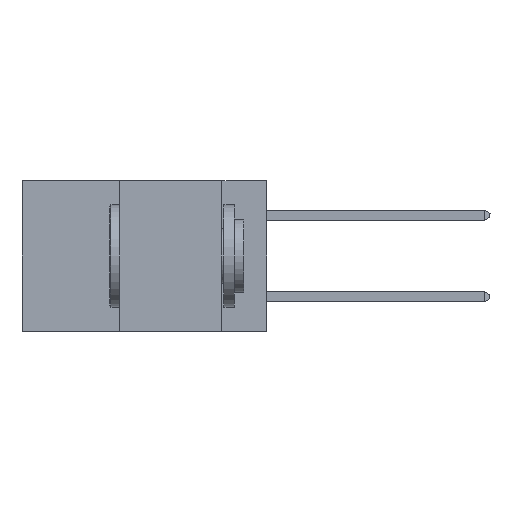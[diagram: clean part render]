
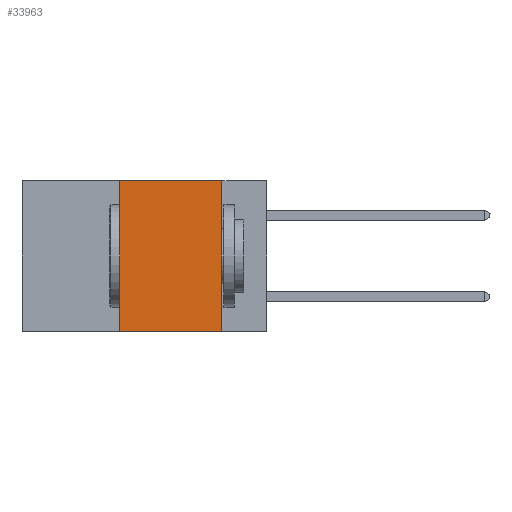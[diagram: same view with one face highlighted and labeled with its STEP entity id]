
A CAD part, left-side view. The second image highlights one B-rep face of the part: STEP entity #33963.
In plain terms, the highlighted planar face has unit normal (-1, 0, 0).
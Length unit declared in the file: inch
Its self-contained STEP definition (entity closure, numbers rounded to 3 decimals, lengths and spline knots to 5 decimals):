
#329 = CARTESIAN_POINT ( 'NONE',  ( 0., 0.6, 0. ) ) ;
#788 = DIRECTION ( 'NONE',  ( 0., 0., 1. ) ) ;
#1015 = CARTESIAN_POINT ( 'NONE',  ( 0., 0.6, 0. ) ) ;
#2139 = CARTESIAN_POINT ( 'NONE',  ( 0., 0.11, -0.37 ) ) ;
#2255 = LINE ( 'NONE', #22179, #9392 ) ;
#3191 = DIRECTION ( 'NONE',  ( 0., -1., 0. ) ) ;
#6124 = DIRECTION ( 'NONE',  ( 0., -1., 0. ) ) ;
#6449 = PLANE ( 'NONE',  #34314 ) ;
#6854 = ORIENTED_EDGE ( 'NONE', *, *, #11763, .F. ) ;
#8208 = EDGE_LOOP ( 'NONE', ( #16887, #12292, #6854, #29658 ) ) ;
#8418 = FACE_OUTER_BOUND ( 'NONE', #8208, .T. ) ;
#8874 = CARTESIAN_POINT ( 'NONE',  ( 0., 0.36, -0.37 ) ) ;
#9163 = DIRECTION ( 'NONE',  ( 1., 0., 0. ) ) ;
#9392 = VECTOR ( 'NONE', #788, 39.37008 ) ;
#10260 = LINE ( 'NONE', #329, #15704 ) ;
#11763 = EDGE_CURVE ( 'NONE', #21095, #29034, #2255, .T. ) ;
#11818 = LINE ( 'NONE', #25637, #25072 ) ;
#12292 = ORIENTED_EDGE ( 'NONE', *, *, #27931, .F. ) ;
#14019 = VECTOR ( 'NONE', #6124, 39.37008 ) ;
#14948 = VERTEX_POINT ( 'NONE', #26959 ) ;
#15704 = VECTOR ( 'NONE', #3191, 39.37008 ) ;
#15871 = VERTEX_POINT ( 'NONE', #2139 ) ;
#16887 = ORIENTED_EDGE ( 'NONE', *, *, #19575, .F. ) ;
#19575 = EDGE_CURVE ( 'NONE', #14948, #15871, #11818, .T. ) ;
#21095 = VERTEX_POINT ( 'NONE', #8874 ) ;
#22083 = CARTESIAN_POINT ( 'NONE',  ( 0., 0.6, -0.37 ) ) ;
#22179 = CARTESIAN_POINT ( 'NONE',  ( 0., 0.36, 0. ) ) ;
#25072 = VECTOR ( 'NONE', #30793, 39.37008 ) ;
#25637 = CARTESIAN_POINT ( 'NONE',  ( 0., 0.11, 0. ) ) ;
#26959 = CARTESIAN_POINT ( 'NONE',  ( 0., 0.11, 0. ) ) ;
#27678 = DIRECTION ( 'NONE',  ( 0., 0., -1. ) ) ;
#27931 = EDGE_CURVE ( 'NONE', #29034, #14948, #10260, .T. ) ;
#27991 = EDGE_CURVE ( 'NONE', #21095, #15871, #34240, .T. ) ;
#29034 = VERTEX_POINT ( 'NONE', #31981 ) ;
#29658 = ORIENTED_EDGE ( 'NONE', *, *, #27991, .T. ) ;
#30793 = DIRECTION ( 'NONE',  ( 0., 0., -1. ) ) ;
#31981 = CARTESIAN_POINT ( 'NONE',  ( 0., 0.36, 0. ) ) ;
#33963 = ADVANCED_FACE ( 'NONE', ( #8418 ), #6449, .F. ) ;
#34240 = LINE ( 'NONE', #22083, #14019 ) ;
#34314 = AXIS2_PLACEMENT_3D ( 'NONE', #1015, #9163, #27678 ) ;
